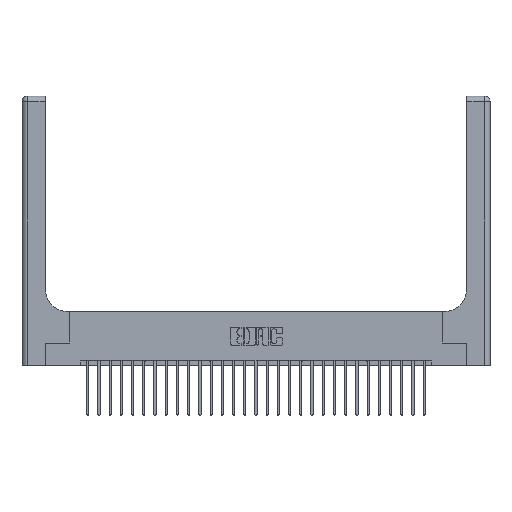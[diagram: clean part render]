
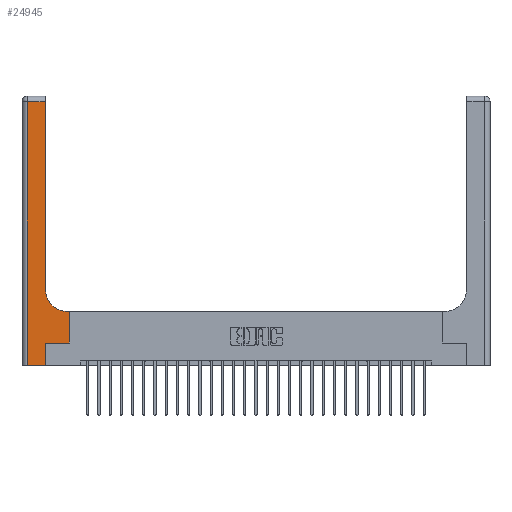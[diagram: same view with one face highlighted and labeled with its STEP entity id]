
A CAD part, top view. The second image highlights one B-rep face of the part: STEP entity #24945.
In plain terms, the highlighted planar face has unit normal (0, 0, 1).
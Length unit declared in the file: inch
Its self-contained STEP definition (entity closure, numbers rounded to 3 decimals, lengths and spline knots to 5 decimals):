
#379 = CIRCLE ( 'NONE', #3927, 0.25 ) ;
#829 = ORIENTED_EDGE ( 'NONE', *, *, #14406, .T. ) ;
#847 = AXIS2_PLACEMENT_3D ( 'NONE', #17700, #26691, #5374 ) ;
#1229 = FACE_OUTER_BOUND ( 'NONE', #13329, .T. ) ;
#1631 = EDGE_CURVE ( 'NONE', #20322, #2990, #13299, .T. ) ;
#1776 = VERTEX_POINT ( 'NONE', #8161 ) ;
#2080 = VERTEX_POINT ( 'NONE', #26820 ) ;
#2192 = DIRECTION ( 'NONE',  ( -1., 0., 0. ) ) ;
#2261 = ORIENTED_EDGE ( 'NONE', *, *, #26938, .T. ) ;
#2923 = LINE ( 'NONE', #22288, #11542 ) ;
#2977 = EDGE_CURVE ( 'NONE', #24937, #1776, #3363, .T. ) ;
#2990 = VERTEX_POINT ( 'NONE', #24278 ) ;
#3165 = PLANE ( 'NONE',  #847 ) ;
#3363 = LINE ( 'NONE', #20106, #9092 ) ;
#3927 = AXIS2_PLACEMENT_3D ( 'NONE', #13989, #26175, #13584 ) ;
#4017 = CARTESIAN_POINT ( 'NONE',  ( 0.06, 2.94, 0.37 ) ) ;
#4528 = CARTESIAN_POINT ( 'NONE',  ( 0.26, 0.6, 0.37 ) ) ;
#5374 = DIRECTION ( 'NONE',  ( -1., 0., 0. ) ) ;
#6277 = VERTEX_POINT ( 'NONE', #8041 ) ;
#6337 = LINE ( 'NONE', #4528, #13972 ) ;
#7113 = CARTESIAN_POINT ( 'NONE',  ( 0.51, 0.6, 0.37 ) ) ;
#7627 = ORIENTED_EDGE ( 'NONE', *, *, #22081, .T. ) ;
#7651 = DIRECTION ( 'NONE',  ( 0., 1., 0. ) ) ;
#8041 = CARTESIAN_POINT ( 'NONE',  ( 0.265, 0., 0.37 ) ) ;
#8161 = CARTESIAN_POINT ( 'NONE',  ( 0.528, 0.6, 0.37 ) ) ;
#8185 = VERTEX_POINT ( 'NONE', #25706 ) ;
#8949 = CARTESIAN_POINT ( 'NONE',  ( 0.26, 3., 0.37 ) ) ;
#9092 = VECTOR ( 'NONE', #7651, 39.37008 ) ;
#9161 = CARTESIAN_POINT ( 'NONE',  ( 0.06, 3., 0.37 ) ) ;
#9898 = ORIENTED_EDGE ( 'NONE', *, *, #17723, .T. ) ;
#11483 = CARTESIAN_POINT ( 'NONE',  ( 0.528, 0.25, 0.37 ) ) ;
#11542 = VECTOR ( 'NONE', #13440, 39.37008 ) ;
#11666 = CARTESIAN_POINT ( 'NONE',  ( 0.26, 0.85, 0.37 ) ) ;
#13299 = LINE ( 'NONE', #9161, #18829 ) ;
#13329 = EDGE_LOOP ( 'NONE', ( #19416, #2261, #19788, #9898, #23245, #829, #25972, #7627, #17530 ) ) ;
#13349 = VERTEX_POINT ( 'NONE', #11666 ) ;
#13440 = DIRECTION ( 'NONE',  ( -1., 0., 0. ) ) ;
#13584 = DIRECTION ( 'NONE',  ( 1., 0., 0. ) ) ;
#13972 = VECTOR ( 'NONE', #2192, 39.37008 ) ;
#13989 = CARTESIAN_POINT ( 'NONE',  ( 0.51, 0.85, 0.37 ) ) ;
#14406 = EDGE_CURVE ( 'NONE', #2080, #24937, #21635, .T. ) ;
#17530 = ORIENTED_EDGE ( 'NONE', *, *, #20198, .T. ) ;
#17700 = CARTESIAN_POINT ( 'NONE',  ( 0., 3., 0.37 ) ) ;
#17723 = EDGE_CURVE ( 'NONE', #2990, #6277, #22313, .T. ) ;
#17855 = LINE ( 'NONE', #19509, #19744 ) ;
#17990 = VECTOR ( 'NONE', #23848, 39.37008 ) ;
#18037 = EDGE_CURVE ( 'NONE', #6277, #2080, #17855, .T. ) ;
#18829 = VECTOR ( 'NONE', #25888, 39.37008 ) ;
#19416 = ORIENTED_EDGE ( 'NONE', *, *, #23616, .T. ) ;
#19509 = CARTESIAN_POINT ( 'NONE',  ( 0.265, 0., 0.37 ) ) ;
#19734 = DIRECTION ( 'NONE',  ( 0., 1., 0. ) ) ;
#19744 = VECTOR ( 'NONE', #26303, 39.37008 ) ;
#19788 = ORIENTED_EDGE ( 'NONE', *, *, #1631, .T. ) ;
#20106 = CARTESIAN_POINT ( 'NONE',  ( 0.528, 0.25, 0.37 ) ) ;
#20198 = EDGE_CURVE ( 'NONE', #25179, #13349, #379, .T. ) ;
#20322 = VERTEX_POINT ( 'NONE', #4017 ) ;
#20372 = CARTESIAN_POINT ( 'NONE',  ( 0., 0., 0.37 ) ) ;
#20502 = DIRECTION ( 'NONE',  ( 1., 0., 0. ) ) ;
#20833 = CARTESIAN_POINT ( 'NONE',  ( 0.265, 0.25, 0.37 ) ) ;
#21635 = LINE ( 'NONE', #20833, #17990 ) ;
#21674 = LINE ( 'NONE', #8949, #22756 ) ;
#22081 = EDGE_CURVE ( 'NONE', #1776, #25179, #6337, .T. ) ;
#22288 = CARTESIAN_POINT ( 'NONE',  ( 0., 2.94, 0.37 ) ) ;
#22313 = LINE ( 'NONE', #20372, #22397 ) ;
#22397 = VECTOR ( 'NONE', #20502, 39.37008 ) ;
#22756 = VECTOR ( 'NONE', #19734, 39.37008 ) ;
#23245 = ORIENTED_EDGE ( 'NONE', *, *, #18037, .T. ) ;
#23616 = EDGE_CURVE ( 'NONE', #13349, #8185, #21674, .T. ) ;
#23848 = DIRECTION ( 'NONE',  ( 1., 0., 0. ) ) ;
#24278 = CARTESIAN_POINT ( 'NONE',  ( 0.06, 0., 0.37 ) ) ;
#24937 = VERTEX_POINT ( 'NONE', #11483 ) ;
#24945 = ADVANCED_FACE ( 'NONE', ( #1229 ), #3165, .F. ) ;
#25179 = VERTEX_POINT ( 'NONE', #7113 ) ;
#25706 = CARTESIAN_POINT ( 'NONE',  ( 0.26, 2.94, 0.37 ) ) ;
#25888 = DIRECTION ( 'NONE',  ( 0., -1., 0. ) ) ;
#25972 = ORIENTED_EDGE ( 'NONE', *, *, #2977, .T. ) ;
#26175 = DIRECTION ( 'NONE',  ( 0., 0., -1. ) ) ;
#26303 = DIRECTION ( 'NONE',  ( 0., 1., 0. ) ) ;
#26691 = DIRECTION ( 'NONE',  ( 0., 0., -1. ) ) ;
#26820 = CARTESIAN_POINT ( 'NONE',  ( 0.265, 0.25, 0.37 ) ) ;
#26938 = EDGE_CURVE ( 'NONE', #8185, #20322, #2923, .T. ) ;
